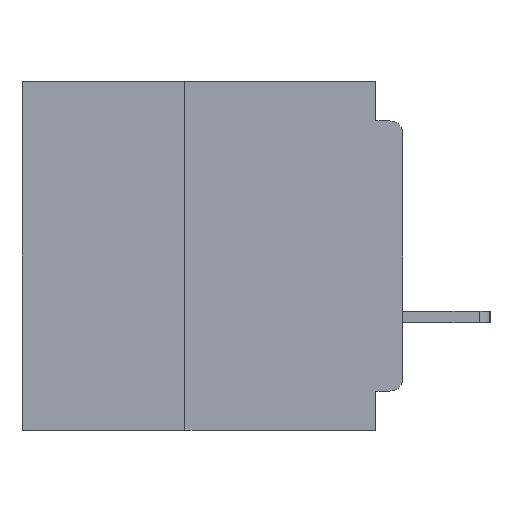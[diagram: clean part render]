
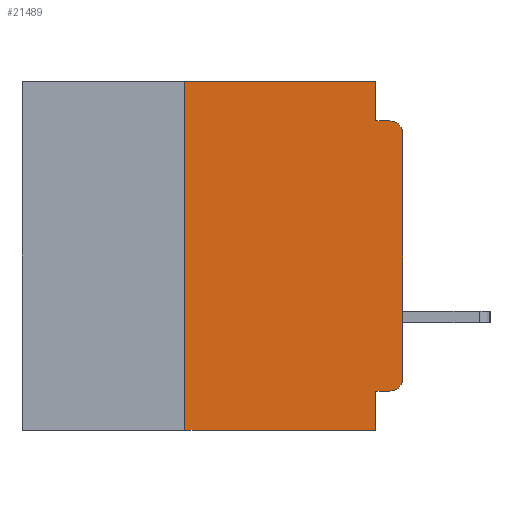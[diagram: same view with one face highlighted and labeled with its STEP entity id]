
A CAD part, left-side view. The second image highlights one B-rep face of the part: STEP entity #21489.
In plain terms, the highlighted planar face has unit normal (-1, 0, 0).
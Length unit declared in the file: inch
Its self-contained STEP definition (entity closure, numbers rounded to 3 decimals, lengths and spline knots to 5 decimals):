
#1051 = LINE ( 'NONE', #22812, #43096 ) ;
#1158 = ORIENTED_EDGE ( 'NONE', *, *, #5935, .F. ) ;
#1288 = VERTEX_POINT ( 'NONE', #51138 ) ;
#1394 = DIRECTION ( 'NONE',  ( 0., 0., 1. ) ) ;
#1782 = VECTOR ( 'NONE', #41521, 39.37008 ) ;
#2159 = EDGE_CURVE ( 'NONE', #39176, #11835, #20056, .T. ) ;
#2683 = ORIENTED_EDGE ( 'NONE', *, *, #2159, .T. ) ;
#2753 = CARTESIAN_POINT ( 'NONE',  ( 0., 0.015, -0.355 ) ) ;
#3715 = LINE ( 'NONE', #25233, #12088 ) ;
#4056 = EDGE_CURVE ( 'NONE', #26099, #25801, #38214, .T. ) ;
#4484 = AXIS2_PLACEMENT_3D ( 'NONE', #27126, #39382, #15105 ) ;
#5396 = ORIENTED_EDGE ( 'NONE', *, *, #11812, .F. ) ;
#5935 = EDGE_CURVE ( 'NONE', #1288, #50240, #3715, .T. ) ;
#6718 = LINE ( 'NONE', #23055, #17597 ) ;
#6965 = CARTESIAN_POINT ( 'NONE',  ( 0., 0.015, -0.06 ) ) ;
#7808 = EDGE_CURVE ( 'NONE', #39176, #10143, #6718, .T. ) ;
#9114 = DIRECTION ( 'NONE',  ( 0., -1., 0. ) ) ;
#9251 = VECTOR ( 'NONE', #13071, 39.37008 ) ;
#10143 = VERTEX_POINT ( 'NONE', #35286 ) ;
#11104 = DIRECTION ( 'NONE',  ( 0., 0., -1. ) ) ;
#11174 = EDGE_CURVE ( 'NONE', #23647, #26099, #12779, .T. ) ;
#11434 = DIRECTION ( 'NONE',  ( 0., -1., 0. ) ) ;
#11599 = EDGE_CURVE ( 'NONE', #27680, #11835, #34283, .T. ) ;
#11812 = EDGE_CURVE ( 'NONE', #23647, #27680, #16592, .T. ) ;
#11835 = VERTEX_POINT ( 'NONE', #30846 ) ;
#12088 = VECTOR ( 'NONE', #9114, 39.37008 ) ;
#12779 = CIRCLE ( 'NONE', #28345, 0.015 ) ;
#13071 = DIRECTION ( 'NONE',  ( 0., -1., 0. ) ) ;
#14371 = DIRECTION ( 'NONE',  ( 0., 1., 0. ) ) ;
#14784 = CARTESIAN_POINT ( 'NONE',  ( 0., 0.015, -0.34 ) ) ;
#15017 = CIRCLE ( 'NONE', #51103, 0.015 ) ;
#15105 = DIRECTION ( 'NONE',  ( 0., 0., -1. ) ) ;
#16592 = LINE ( 'NONE', #50871, #45193 ) ;
#17597 = VECTOR ( 'NONE', #27157, 39.37008 ) ;
#18866 = DIRECTION ( 'NONE',  ( 0., 0., -1. ) ) ;
#19011 = PLANE ( 'NONE',  #4484 ) ;
#20056 = LINE ( 'NONE', #29190, #9251 ) ;
#21123 = VECTOR ( 'NONE', #11434, 39.37008 ) ;
#21131 = CARTESIAN_POINT ( 'NONE',  ( 0., 0.031, -0.355 ) ) ;
#21489 = ADVANCED_FACE ( 'NONE', ( #47402 ), #19011, .F. ) ;
#21840 = ORIENTED_EDGE ( 'NONE', *, *, #27094, .F. ) ;
#22812 = CARTESIAN_POINT ( 'NONE',  ( 0., 0.031, 0. ) ) ;
#23055 = CARTESIAN_POINT ( 'NONE',  ( 0., 0.25, -0.4 ) ) ;
#23083 = EDGE_CURVE ( 'NONE', #10143, #25618, #33199, .T. ) ;
#23647 = VERTEX_POINT ( 'NONE', #2753 ) ;
#24350 = CARTESIAN_POINT ( 'NONE',  ( 0., 0., -0.34 ) ) ;
#25233 = CARTESIAN_POINT ( 'NONE',  ( 0., 0., -0.045 ) ) ;
#25618 = VERTEX_POINT ( 'NONE', #45776 ) ;
#25772 = CARTESIAN_POINT ( 'NONE',  ( 0., 0., 0. ) ) ;
#25801 = VERTEX_POINT ( 'NONE', #26698 ) ;
#25865 = ORIENTED_EDGE ( 'NONE', *, *, #42293, .T. ) ;
#26099 = VERTEX_POINT ( 'NONE', #24350 ) ;
#26698 = CARTESIAN_POINT ( 'NONE',  ( 0., 0., -0.06 ) ) ;
#27094 = EDGE_CURVE ( 'NONE', #25618, #1288, #1051, .T. ) ;
#27126 = CARTESIAN_POINT ( 'NONE',  ( 0., 0.437, 0. ) ) ;
#27157 = DIRECTION ( 'NONE',  ( 0., 0., 1. ) ) ;
#27532 = ORIENTED_EDGE ( 'NONE', *, *, #23083, .F. ) ;
#27680 = VERTEX_POINT ( 'NONE', #21131 ) ;
#28345 = AXIS2_PLACEMENT_3D ( 'NONE', #14784, #43162, #18866 ) ;
#29190 = CARTESIAN_POINT ( 'NONE',  ( 0., 0.437, -0.4 ) ) ;
#30846 = CARTESIAN_POINT ( 'NONE',  ( 0., 0.031, -0.4 ) ) ;
#33199 = LINE ( 'NONE', #48013, #21123 ) ;
#34283 = LINE ( 'NONE', #37424, #1782 ) ;
#35286 = CARTESIAN_POINT ( 'NONE',  ( 0., 0.25, 0. ) ) ;
#35400 = DIRECTION ( 'NONE',  ( -1., 0., 0. ) ) ;
#36334 = ORIENTED_EDGE ( 'NONE', *, *, #11599, .F. ) ;
#37424 = CARTESIAN_POINT ( 'NONE',  ( 0., 0.031, -0.4 ) ) ;
#38214 = LINE ( 'NONE', #25772, #49048 ) ;
#39176 = VERTEX_POINT ( 'NONE', #44174 ) ;
#39382 = DIRECTION ( 'NONE',  ( 1., 0., 0. ) ) ;
#41443 = ORIENTED_EDGE ( 'NONE', *, *, #4056, .T. ) ;
#41521 = DIRECTION ( 'NONE',  ( 0., 0., -1. ) ) ;
#42293 = EDGE_CURVE ( 'NONE', #25801, #50240, #15017, .T. ) ;
#43096 = VECTOR ( 'NONE', #51217, 39.37008 ) ;
#43162 = DIRECTION ( 'NONE',  ( -1., 0., 0. ) ) ;
#44174 = CARTESIAN_POINT ( 'NONE',  ( 0., 0.25, -0.4 ) ) ;
#45193 = VECTOR ( 'NONE', #14371, 39.37008 ) ;
#45776 = CARTESIAN_POINT ( 'NONE',  ( 0., 0.031, 0. ) ) ;
#47402 = FACE_OUTER_BOUND ( 'NONE', #48230, .T. ) ;
#48013 = CARTESIAN_POINT ( 'NONE',  ( 0., 0.437, 0. ) ) ;
#48230 = EDGE_LOOP ( 'NONE', ( #41443, #25865, #1158, #21840, #27532, #49615, #2683, #36334, #5396, #50994 ) ) ;
#49048 = VECTOR ( 'NONE', #1394, 39.37008 ) ;
#49615 = ORIENTED_EDGE ( 'NONE', *, *, #7808, .F. ) ;
#50240 = VERTEX_POINT ( 'NONE', #50979 ) ;
#50871 = CARTESIAN_POINT ( 'NONE',  ( 0., 0., -0.355 ) ) ;
#50979 = CARTESIAN_POINT ( 'NONE',  ( 0., 0.015, -0.045 ) ) ;
#50994 = ORIENTED_EDGE ( 'NONE', *, *, #11174, .T. ) ;
#51103 = AXIS2_PLACEMENT_3D ( 'NONE', #6965, #35400, #11104 ) ;
#51138 = CARTESIAN_POINT ( 'NONE',  ( 0., 0.031, -0.045 ) ) ;
#51217 = DIRECTION ( 'NONE',  ( 0., 0., -1. ) ) ;
